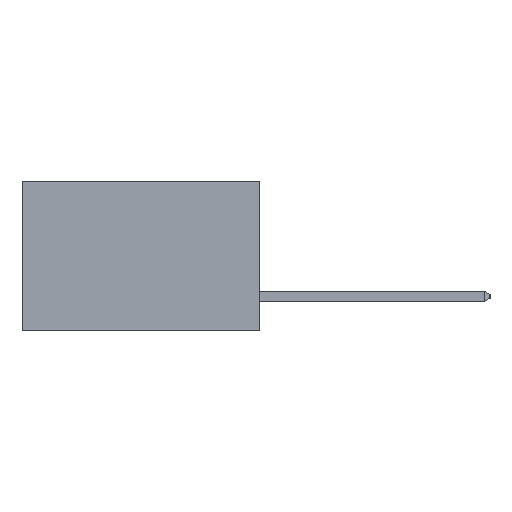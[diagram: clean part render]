
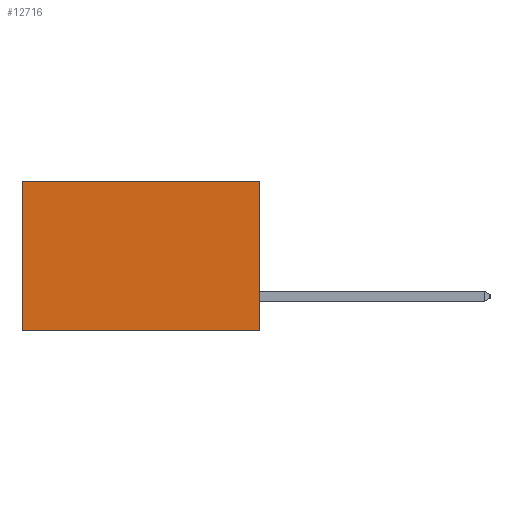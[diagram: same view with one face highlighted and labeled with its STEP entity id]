
A CAD part, left-side view. The second image highlights one B-rep face of the part: STEP entity #12716.
In plain terms, the highlighted planar face has unit normal (-1, 0, 0).
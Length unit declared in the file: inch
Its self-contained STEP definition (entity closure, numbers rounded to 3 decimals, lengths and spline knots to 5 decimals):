
#1535 = CARTESIAN_POINT ( 'NONE',  ( 0.277, 0.59, -0.37 ) ) ;
#1682 = LINE ( 'NONE', #11141, #11006 ) ;
#1687 = CARTESIAN_POINT ( 'NONE',  ( 0.277, 0.59, 0. ) ) ;
#1816 = VECTOR ( 'NONE', #14559, 39.37008 ) ;
#2305 = VERTEX_POINT ( 'NONE', #1687 ) ;
#3536 = EDGE_CURVE ( 'NONE', #17317, #11043, #8827, .T. ) ;
#3602 = PLANE ( 'NONE',  #8715 ) ;
#4288 = EDGE_CURVE ( 'NONE', #2305, #5082, #1682, .T. ) ;
#4715 = CARTESIAN_POINT ( 'NONE',  ( 0.277, 0., -0.37 ) ) ;
#5031 = CARTESIAN_POINT ( 'NONE',  ( 0.277, 0., 0. ) ) ;
#5082 = VERTEX_POINT ( 'NONE', #1535 ) ;
#5481 = DIRECTION ( 'NONE',  ( 0., 0., -1. ) ) ;
#6621 = LINE ( 'NONE', #4715, #20268 ) ;
#7445 = CARTESIAN_POINT ( 'NONE',  ( 0.277, 0., 0. ) ) ;
#8715 = AXIS2_PLACEMENT_3D ( 'NONE', #14515, #16329, #5481 ) ;
#8827 = LINE ( 'NONE', #20770, #13522 ) ;
#9419 = FACE_OUTER_BOUND ( 'NONE', #14608, .T. ) ;
#11006 = VECTOR ( 'NONE', #11096, 39.37008 ) ;
#11043 = VERTEX_POINT ( 'NONE', #11154 ) ;
#11096 = DIRECTION ( 'NONE',  ( 0., 0., -1. ) ) ;
#11123 = LINE ( 'NONE', #7445, #1816 ) ;
#11141 = CARTESIAN_POINT ( 'NONE',  ( 0.277, 0.59, -0.37 ) ) ;
#11154 = CARTESIAN_POINT ( 'NONE',  ( 0.277, 0., -0.37 ) ) ;
#12716 = ADVANCED_FACE ( 'NONE', ( #9419 ), #3602, .F. ) ;
#13522 = VECTOR ( 'NONE', #20684, 39.37008 ) ;
#14515 = CARTESIAN_POINT ( 'NONE',  ( 0.277, 0., -0.37 ) ) ;
#14559 = DIRECTION ( 'NONE',  ( 0., 1., 0. ) ) ;
#14608 = EDGE_LOOP ( 'NONE', ( #21794, #21066, #21040, #20898 ) ) ;
#14656 = EDGE_CURVE ( 'NONE', #17317, #2305, #11123, .T. ) ;
#16329 = DIRECTION ( 'NONE',  ( 1., 0., 0. ) ) ;
#17317 = VERTEX_POINT ( 'NONE', #5031 ) ;
#20268 = VECTOR ( 'NONE', #22559, 39.37008 ) ;
#20684 = DIRECTION ( 'NONE',  ( 0., 0., -1. ) ) ;
#20770 = CARTESIAN_POINT ( 'NONE',  ( 0.277, 0., -0.37 ) ) ;
#20898 = ORIENTED_EDGE ( 'NONE', *, *, #14656, .T. ) ;
#21040 = ORIENTED_EDGE ( 'NONE', *, *, #3536, .F. ) ;
#21066 = ORIENTED_EDGE ( 'NONE', *, *, #23139, .F. ) ;
#21794 = ORIENTED_EDGE ( 'NONE', *, *, #4288, .T. ) ;
#22559 = DIRECTION ( 'NONE',  ( 0., 1., 0. ) ) ;
#23139 = EDGE_CURVE ( 'NONE', #11043, #5082, #6621, .T. ) ;
